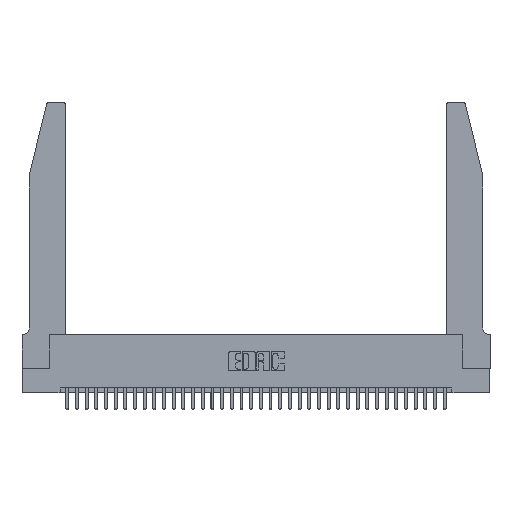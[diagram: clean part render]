
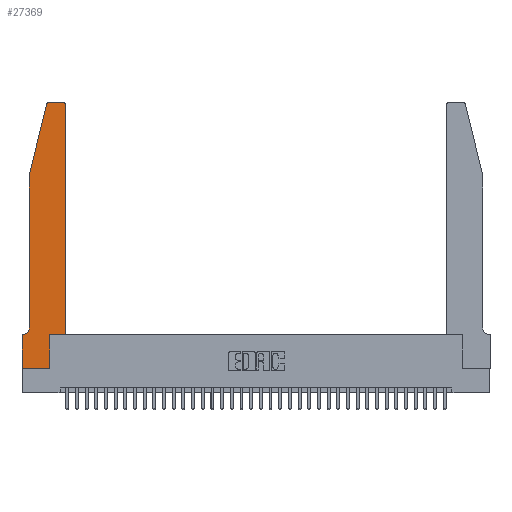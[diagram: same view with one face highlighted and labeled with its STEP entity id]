
A CAD part, top view. The second image highlights one B-rep face of the part: STEP entity #27369.
In plain terms, the highlighted planar face has unit normal (0, 0, 1).
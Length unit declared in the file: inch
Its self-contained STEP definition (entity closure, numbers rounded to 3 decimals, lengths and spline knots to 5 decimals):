
#810 = ORIENTED_EDGE ( 'NONE', *, *, #16064, .T. ) ;
#1501 = CARTESIAN_POINT ( 'NONE',  ( 0.2865, 0., 0.37 ) ) ;
#1629 = EDGE_CURVE ( 'NONE', #5479, #6710, #2720, .T. ) ;
#1752 = CARTESIAN_POINT ( 'NONE',  ( 0.4505, 0.35, 0.37 ) ) ;
#1973 = DIRECTION ( 'NONE',  ( 1., 0., 0. ) ) ;
#2145 = FACE_OUTER_BOUND ( 'NONE', #10114, .T. ) ;
#2720 = LINE ( 'NONE', #13883, #29179 ) ;
#3241 = CARTESIAN_POINT ( 'NONE',  ( 0.0755, 2., 0.37 ) ) ;
#3461 = DIRECTION ( 'NONE',  ( -1., 0., 0. ) ) ;
#3465 = DIRECTION ( 'NONE',  ( 0., 0., 1. ) ) ;
#3504 = EDGE_CURVE ( 'NONE', #32504, #34312, #10490, .T. ) ;
#3805 = EDGE_CURVE ( 'NONE', #35985, #35412, #28134, .T. ) ;
#4634 = CARTESIAN_POINT ( 'NONE',  ( 0.0755, 0.35, 0.37 ) ) ;
#4890 = EDGE_CURVE ( 'NONE', #6710, #32504, #15663, .T. ) ;
#4949 = VECTOR ( 'NONE', #9980, 39.37008 ) ;
#4978 = ORIENTED_EDGE ( 'NONE', *, *, #10328, .T. ) ;
#5345 = VERTEX_POINT ( 'NONE', #27641 ) ;
#5464 = ORIENTED_EDGE ( 'NONE', *, *, #15135, .T. ) ;
#5479 = VERTEX_POINT ( 'NONE', #33442 ) ;
#5785 = CARTESIAN_POINT ( 'NONE',  ( 0.2605, 2.75, 0.37 ) ) ;
#6301 = DIRECTION ( 'NONE',  ( 1., 0., 0. ) ) ;
#6710 = VERTEX_POINT ( 'NONE', #3241 ) ;
#7288 = CARTESIAN_POINT ( 'NONE',  ( 0.0055, 0.35, 0.37 ) ) ;
#8041 = ORIENTED_EDGE ( 'NONE', *, *, #4890, .T. ) ;
#8550 = VERTEX_POINT ( 'NONE', #33240 ) ;
#8667 = LINE ( 'NONE', #14683, #31548 ) ;
#9092 = DIRECTION ( 'NONE',  ( -1., 0., 0. ) ) ;
#9773 = AXIS2_PLACEMENT_3D ( 'NONE', #21828, #33190, #24447 ) ;
#9839 = AXIS2_PLACEMENT_3D ( 'NONE', #32546, #18872, #1973 ) ;
#9980 = DIRECTION ( 'NONE',  ( 0., 1., 0. ) ) ;
#10114 = EDGE_LOOP ( 'NONE', ( #22618, #35989, #28849, #8041, #25222, #4978, #5464, #36159, #20079, #15927, #15936, #810 ) ) ;
#10328 = EDGE_CURVE ( 'NONE', #34312, #36130, #29834, .T. ) ;
#10490 = CIRCLE ( 'NONE', #24445, 0.07 ) ;
#10768 = EDGE_CURVE ( 'NONE', #5345, #26690, #8667, .T. ) ;
#10893 = VECTOR ( 'NONE', #31654, 39.37008 ) ;
#11034 = CARTESIAN_POINT ( 'NONE',  ( 0.2865, 0.35, 0.37 ) ) ;
#11736 = EDGE_CURVE ( 'NONE', #8550, #35300, #18688, .T. ) ;
#11909 = CARTESIAN_POINT ( 'NONE',  ( 0.0755, 2., 0.37 ) ) ;
#12727 = CARTESIAN_POINT ( 'NONE',  ( 0.4205, 2.75, 0.37 ) ) ;
#13167 = EDGE_CURVE ( 'NONE', #26690, #27418, #25673, .T. ) ;
#13430 = LINE ( 'NONE', #34166, #18695 ) ;
#13883 = CARTESIAN_POINT ( 'NONE',  ( 0.0755, 2., 0.37 ) ) ;
#14683 = CARTESIAN_POINT ( 'NONE',  ( 0.4505, 0.35, 0.37 ) ) ;
#15009 = DIRECTION ( 'NONE',  ( 0., 1., 0. ) ) ;
#15135 = EDGE_CURVE ( 'NONE', #36130, #8550, #13430, .T. ) ;
#15663 = LINE ( 'NONE', #11909, #10893 ) ;
#15927 = ORIENTED_EDGE ( 'NONE', *, *, #10768, .T. ) ;
#15936 = ORIENTED_EDGE ( 'NONE', *, *, #13167, .T. ) ;
#16064 = EDGE_CURVE ( 'NONE', #27418, #35985, #34544, .T. ) ;
#16854 = EDGE_CURVE ( 'NONE', #35300, #5345, #35386, .T. ) ;
#17783 = VECTOR ( 'NONE', #26489, 39.37008 ) ;
#17888 = EDGE_CURVE ( 'NONE', #35412, #5479, #31741, .T. ) ;
#18570 = DIRECTION ( 'NONE',  ( -1., 0., 0. ) ) ;
#18688 = LINE ( 'NONE', #29083, #17783 ) ;
#18695 = VECTOR ( 'NONE', #25774, 39.37008 ) ;
#18872 = DIRECTION ( 'NONE',  ( 0., 0., 1. ) ) ;
#19004 = CARTESIAN_POINT ( 'NONE',  ( 0.4505, 2.72, 0.37 ) ) ;
#19783 = CARTESIAN_POINT ( 'NONE',  ( 0., 0.35, 0.37 ) ) ;
#20039 = DIRECTION ( 'NONE',  ( 0., 0., -1. ) ) ;
#20079 = ORIENTED_EDGE ( 'NONE', *, *, #16854, .T. ) ;
#20137 = VECTOR ( 'NONE', #9092, 39.37008 ) ;
#21828 = CARTESIAN_POINT ( 'NONE',  ( 0., 0.35, 0.37 ) ) ;
#22549 = CARTESIAN_POINT ( 'NONE',  ( 0.284, 2.72, 0.37 ) ) ;
#22618 = ORIENTED_EDGE ( 'NONE', *, *, #3805, .T. ) ;
#24445 = AXIS2_PLACEMENT_3D ( 'NONE', #28782, #20039, #3461 ) ;
#24447 = DIRECTION ( 'NONE',  ( 1., 0., 0. ) ) ;
#25096 = AXIS2_PLACEMENT_3D ( 'NONE', #22549, #3465, #6301 ) ;
#25222 = ORIENTED_EDGE ( 'NONE', *, *, #3504, .T. ) ;
#25673 = LINE ( 'NONE', #34113, #29624 ) ;
#25774 = DIRECTION ( 'NONE',  ( 0., -1., 0. ) ) ;
#26195 = DIRECTION ( 'NONE',  ( 1., 0., 0. ) ) ;
#26489 = DIRECTION ( 'NONE',  ( 1., 0., 0. ) ) ;
#26690 = VERTEX_POINT ( 'NONE', #1752 ) ;
#27369 = ADVANCED_FACE ( 'NONE', ( #2145 ), #33060, .T. ) ;
#27418 = VERTEX_POINT ( 'NONE', #19004 ) ;
#27641 = CARTESIAN_POINT ( 'NONE',  ( 0.2865, 0.35, 0.37 ) ) ;
#27963 = DIRECTION ( 'NONE',  ( -0.239, -0.971, 0. ) ) ;
#28134 = LINE ( 'NONE', #5785, #20137 ) ;
#28782 = CARTESIAN_POINT ( 'NONE',  ( 0.0055, 0.42, 0.37 ) ) ;
#28849 = ORIENTED_EDGE ( 'NONE', *, *, #1629, .T. ) ;
#29083 = CARTESIAN_POINT ( 'NONE',  ( 0., 0., 0.37 ) ) ;
#29179 = VECTOR ( 'NONE', #27963, 39.37008 ) ;
#29624 = VECTOR ( 'NONE', #15009, 39.37008 ) ;
#29776 = CARTESIAN_POINT ( 'NONE',  ( 0.284, 2.75, 0.37 ) ) ;
#29834 = LINE ( 'NONE', #4634, #34666 ) ;
#31548 = VECTOR ( 'NONE', #26195, 39.37008 ) ;
#31654 = DIRECTION ( 'NONE',  ( 0., -1., 0. ) ) ;
#31741 = CIRCLE ( 'NONE', #25096, 0.03 ) ;
#32504 = VERTEX_POINT ( 'NONE', #35818 ) ;
#32546 = CARTESIAN_POINT ( 'NONE',  ( 0.4205, 2.72, 0.37 ) ) ;
#33060 = PLANE ( 'NONE',  #9773 ) ;
#33190 = DIRECTION ( 'NONE',  ( 0., 0., 1. ) ) ;
#33240 = CARTESIAN_POINT ( 'NONE',  ( 0., 0., 0.37 ) ) ;
#33442 = CARTESIAN_POINT ( 'NONE',  ( 0.25487, 2.72718, 0.37 ) ) ;
#34113 = CARTESIAN_POINT ( 'NONE',  ( 0.4505, 0.35, 0.37 ) ) ;
#34166 = CARTESIAN_POINT ( 'NONE',  ( 0., 0., 0.37 ) ) ;
#34312 = VERTEX_POINT ( 'NONE', #7288 ) ;
#34544 = CIRCLE ( 'NONE', #9839, 0.03 ) ;
#34666 = VECTOR ( 'NONE', #18570, 39.37008 ) ;
#35300 = VERTEX_POINT ( 'NONE', #1501 ) ;
#35386 = LINE ( 'NONE', #11034, #4949 ) ;
#35412 = VERTEX_POINT ( 'NONE', #29776 ) ;
#35818 = CARTESIAN_POINT ( 'NONE',  ( 0.0755, 0.42, 0.37 ) ) ;
#35985 = VERTEX_POINT ( 'NONE', #12727 ) ;
#35989 = ORIENTED_EDGE ( 'NONE', *, *, #17888, .T. ) ;
#36130 = VERTEX_POINT ( 'NONE', #19783 ) ;
#36159 = ORIENTED_EDGE ( 'NONE', *, *, #11736, .T. ) ;
